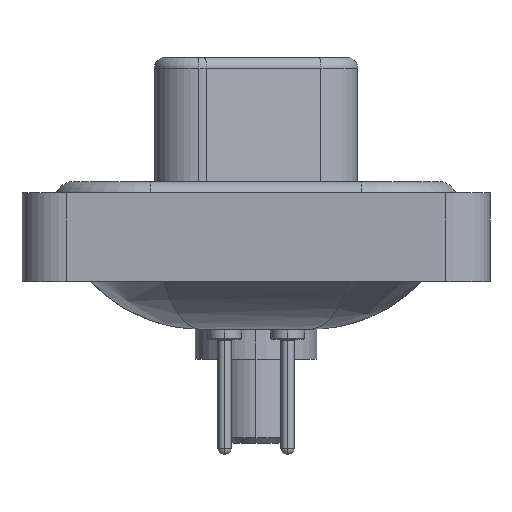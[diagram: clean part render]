
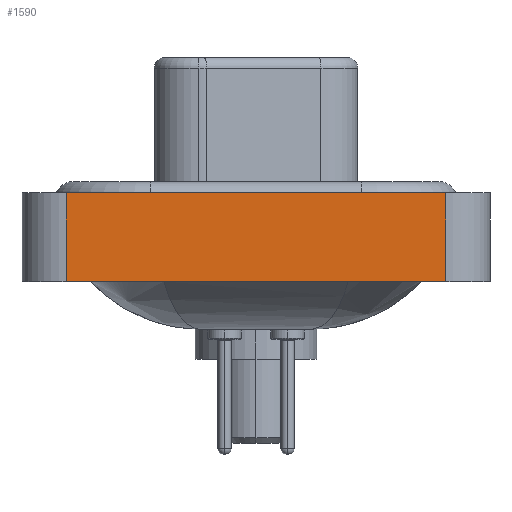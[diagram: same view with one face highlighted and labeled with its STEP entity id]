
A CAD part, left-side view. The second image highlights one B-rep face of the part: STEP entity #1590.
In plain terms, the highlighted planar face has unit normal (-1, 0, 0).
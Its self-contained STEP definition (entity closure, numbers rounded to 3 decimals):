
#504 = FACE_OUTER_BOUND ( 'NONE', #11296, .T. ) ;
#872 = DIRECTION ( 'NONE',  ( 0., -1., 0. ) ) ;
#1590 = ADVANCED_FACE ( 'NONE', ( #504 ), #2933, .T. ) ;
#2264 = CARTESIAN_POINT ( 'NONE',  ( -7.3, 8.55, -3.6 ) ) ;
#2517 = DIRECTION ( 'NONE',  ( 0., 0., 1. ) ) ;
#2789 = CARTESIAN_POINT ( 'NONE',  ( -7.3, 8.55, -3.6 ) ) ;
#2814 = VERTEX_POINT ( 'NONE', #16278 ) ;
#2822 = CARTESIAN_POINT ( 'NONE',  ( -7.3, -8.55, -3.6 ) ) ;
#2933 = PLANE ( 'NONE',  #6582 ) ;
#3940 = DIRECTION ( 'NONE',  ( 0., 0., 1. ) ) ;
#3988 = VERTEX_POINT ( 'NONE', #2789 ) ;
#4205 = CARTESIAN_POINT ( 'NONE',  ( -7.3, -8.55, -3.6 ) ) ;
#4321 = EDGE_CURVE ( 'NONE', #20745, #2814, #12074, .T. ) ;
#4771 = EDGE_CURVE ( 'NONE', #3988, #5152, #20822, .T. ) ;
#5018 = VECTOR ( 'NONE', #872, 1000. ) ;
#5076 = VECTOR ( 'NONE', #17240, 1000. ) ;
#5152 = VERTEX_POINT ( 'NONE', #20186 ) ;
#5523 = LINE ( 'NONE', #2264, #20370 ) ;
#6222 = EDGE_CURVE ( 'NONE', #3988, #20745, #5523, .T. ) ;
#6582 = AXIS2_PLACEMENT_3D ( 'NONE', #4205, #17340, #2517 ) ;
#7169 = EDGE_CURVE ( 'NONE', #5152, #2814, #9147, .T. ) ;
#9147 = LINE ( 'NONE', #9545, #11002 ) ;
#9545 = CARTESIAN_POINT ( 'NONE',  ( -7.3, -8.55, -3.6 ) ) ;
#10159 = CARTESIAN_POINT ( 'NONE',  ( -7.3, 8.55, 0.4 ) ) ;
#11002 = VECTOR ( 'NONE', #19097, 1000. ) ;
#11296 = EDGE_LOOP ( 'NONE', ( #15537, #12635, #16289, #15465 ) ) ;
#12074 = LINE ( 'NONE', #13879, #5018 ) ;
#12635 = ORIENTED_EDGE ( 'NONE', *, *, #4321, .F. ) ;
#13879 = CARTESIAN_POINT ( 'NONE',  ( -7.3, -8.55, 0.4 ) ) ;
#15465 = ORIENTED_EDGE ( 'NONE', *, *, #4771, .T. ) ;
#15537 = ORIENTED_EDGE ( 'NONE', *, *, #7169, .T. ) ;
#16278 = CARTESIAN_POINT ( 'NONE',  ( -7.3, -8.55, 0.4 ) ) ;
#16289 = ORIENTED_EDGE ( 'NONE', *, *, #6222, .F. ) ;
#17240 = DIRECTION ( 'NONE',  ( 0., -1., 0. ) ) ;
#17340 = DIRECTION ( 'NONE',  ( -1., 0., 0. ) ) ;
#19097 = DIRECTION ( 'NONE',  ( 0., 0., 1. ) ) ;
#20186 = CARTESIAN_POINT ( 'NONE',  ( -7.3, -8.55, -3.6 ) ) ;
#20370 = VECTOR ( 'NONE', #3940, 1000. ) ;
#20745 = VERTEX_POINT ( 'NONE', #10159 ) ;
#20822 = LINE ( 'NONE', #2822, #5076 ) ;
